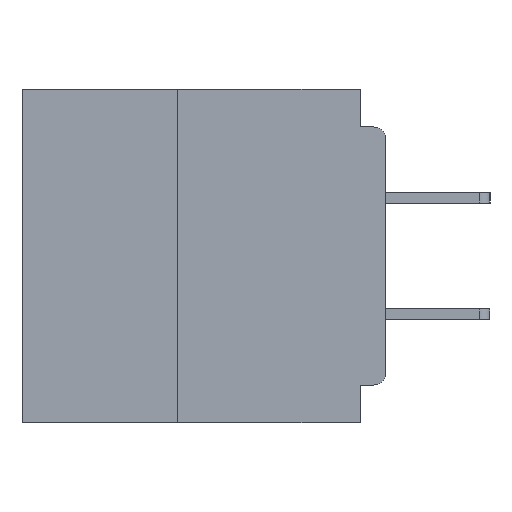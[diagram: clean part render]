
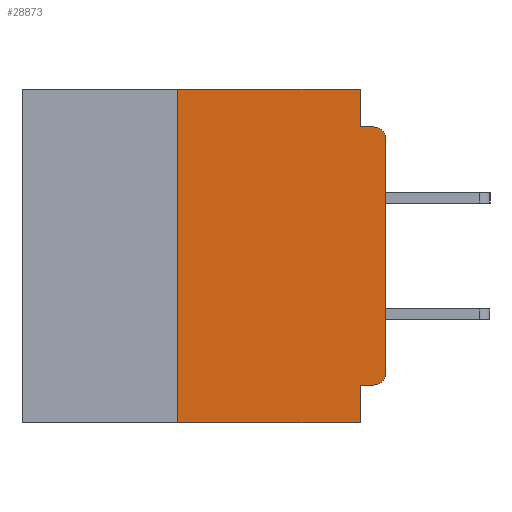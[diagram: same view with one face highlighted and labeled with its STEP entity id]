
A CAD part, left-side view. The second image highlights one B-rep face of the part: STEP entity #28873.
In plain terms, the highlighted planar face has unit normal (-1, 0, 0).
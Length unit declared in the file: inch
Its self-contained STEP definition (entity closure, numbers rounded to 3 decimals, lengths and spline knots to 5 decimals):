
#457 = VECTOR ( 'NONE', #17460, 39.37008 ) ;
#2087 = CARTESIAN_POINT ( 'NONE',  ( 0., 0.25, -0.4 ) ) ;
#2318 = LINE ( 'NONE', #58932, #50608 ) ;
#2635 = VERTEX_POINT ( 'NONE', #54637 ) ;
#4179 = AXIS2_PLACEMENT_3D ( 'NONE', #40658, #12678, #45377 ) ;
#4565 = ORIENTED_EDGE ( 'NONE', *, *, #20370, .T. ) ;
#4714 = LINE ( 'NONE', #22511, #15736 ) ;
#4719 = VERTEX_POINT ( 'NONE', #5902 ) ;
#4881 = LINE ( 'NONE', #22157, #457 ) ;
#5902 = CARTESIAN_POINT ( 'NONE',  ( 0., 0.031, -0.355 ) ) ;
#7995 = CARTESIAN_POINT ( 'NONE',  ( 0., 0.031, 0. ) ) ;
#9453 = ORIENTED_EDGE ( 'NONE', *, *, #44359, .F. ) ;
#9555 = VECTOR ( 'NONE', #11572, 39.37008 ) ;
#9709 = DIRECTION ( 'NONE',  ( -1., 0., 0. ) ) ;
#10058 = LINE ( 'NONE', #37524, #42948 ) ;
#10267 = CARTESIAN_POINT ( 'NONE',  ( 0., 0.031, -0.4 ) ) ;
#10678 = CARTESIAN_POINT ( 'NONE',  ( 0., 0.015, -0.045 ) ) ;
#10918 = DIRECTION ( 'NONE',  ( 0., -1., 0. ) ) ;
#11186 = CARTESIAN_POINT ( 'NONE',  ( 0., 0., -0.34 ) ) ;
#11572 = DIRECTION ( 'NONE',  ( 0., 0., 1. ) ) ;
#11815 = DIRECTION ( 'NONE',  ( 0., 1., 0. ) ) ;
#12678 = DIRECTION ( 'NONE',  ( -1., 0., 0. ) ) ;
#14697 = CIRCLE ( 'NONE', #4179, 0.015 ) ;
#15736 = VECTOR ( 'NONE', #41263, 39.37008 ) ;
#17439 = LINE ( 'NONE', #44492, #54642 ) ;
#17460 = DIRECTION ( 'NONE',  ( 0., -1., 0. ) ) ;
#18369 = DIRECTION ( 'NONE',  ( 1., 0., 0. ) ) ;
#18534 = DIRECTION ( 'NONE',  ( 0., 0., -1. ) ) ;
#19513 = VERTEX_POINT ( 'NONE', #10267 ) ;
#19910 = EDGE_LOOP ( 'NONE', ( #4565, #28558, #40858, #48947, #9453, #22079, #47818, #60266, #43933, #29171 ) ) ;
#20370 = EDGE_CURVE ( 'NONE', #49438, #37737, #2318, .T. ) ;
#22079 = ORIENTED_EDGE ( 'NONE', *, *, #51450, .F. ) ;
#22157 = CARTESIAN_POINT ( 'NONE',  ( 0., 0., -0.045 ) ) ;
#22481 = AXIS2_PLACEMENT_3D ( 'NONE', #37696, #9709, #42407 ) ;
#22511 = CARTESIAN_POINT ( 'NONE',  ( 0., 0.437, 0. ) ) ;
#23654 = VERTEX_POINT ( 'NONE', #10678 ) ;
#24837 = CARTESIAN_POINT ( 'NONE',  ( 0., 0.031, -0.045 ) ) ;
#28186 = EDGE_CURVE ( 'NONE', #37737, #23654, #38001, .T. ) ;
#28558 = ORIENTED_EDGE ( 'NONE', *, *, #28186, .T. ) ;
#28873 = ADVANCED_FACE ( 'NONE', ( #46676 ), #46348, .F. ) ;
#29171 = ORIENTED_EDGE ( 'NONE', *, *, #38684, .T. ) ;
#30952 = VERTEX_POINT ( 'NONE', #34091 ) ;
#30955 = LINE ( 'NONE', #7995, #33883 ) ;
#30957 = VECTOR ( 'NONE', #10918, 39.37008 ) ;
#31080 = DIRECTION ( 'NONE',  ( 0., 0., 1. ) ) ;
#32741 = EDGE_CURVE ( 'NONE', #59971, #19513, #43370, .T. ) ;
#33669 = CARTESIAN_POINT ( 'NONE',  ( 0., 0., -0.06 ) ) ;
#33883 = VECTOR ( 'NONE', #40679, 39.37008 ) ;
#34091 = CARTESIAN_POINT ( 'NONE',  ( 0., 0.25, 0. ) ) ;
#36750 = CARTESIAN_POINT ( 'NONE',  ( 0., 0.437, 0. ) ) ;
#37524 = CARTESIAN_POINT ( 'NONE',  ( 0., 0.031, -0.4 ) ) ;
#37696 = CARTESIAN_POINT ( 'NONE',  ( 0., 0.015, -0.06 ) ) ;
#37737 = VERTEX_POINT ( 'NONE', #33669 ) ;
#38001 = CIRCLE ( 'NONE', #22481, 0.015 ) ;
#38684 = EDGE_CURVE ( 'NONE', #2635, #49438, #14697, .T. ) ;
#40658 = CARTESIAN_POINT ( 'NONE',  ( 0., 0.015, -0.34 ) ) ;
#40679 = DIRECTION ( 'NONE',  ( 0., 0., -1. ) ) ;
#40858 = ORIENTED_EDGE ( 'NONE', *, *, #53920, .F. ) ;
#41263 = DIRECTION ( 'NONE',  ( 0., -1., 0. ) ) ;
#42407 = DIRECTION ( 'NONE',  ( 0., 0., -1. ) ) ;
#42636 = EDGE_CURVE ( 'NONE', #2635, #4719, #17439, .T. ) ;
#42948 = VECTOR ( 'NONE', #18534, 39.37008 ) ;
#43271 = EDGE_CURVE ( 'NONE', #4719, #19513, #10058, .T. ) ;
#43370 = LINE ( 'NONE', #52744, #30957 ) ;
#43933 = ORIENTED_EDGE ( 'NONE', *, *, #42636, .F. ) ;
#44359 = EDGE_CURVE ( 'NONE', #30952, #52330, #4714, .T. ) ;
#44492 = CARTESIAN_POINT ( 'NONE',  ( 0., 0., -0.355 ) ) ;
#45196 = AXIS2_PLACEMENT_3D ( 'NONE', #36750, #18369, #51024 ) ;
#45377 = DIRECTION ( 'NONE',  ( 0., 0., -1. ) ) ;
#46348 = PLANE ( 'NONE',  #45196 ) ;
#46676 = FACE_OUTER_BOUND ( 'NONE', #19910, .T. ) ;
#47665 = CARTESIAN_POINT ( 'NONE',  ( 0., 0.031, 0. ) ) ;
#47818 = ORIENTED_EDGE ( 'NONE', *, *, #32741, .T. ) ;
#48947 = ORIENTED_EDGE ( 'NONE', *, *, #50287, .F. ) ;
#49438 = VERTEX_POINT ( 'NONE', #11186 ) ;
#50287 = EDGE_CURVE ( 'NONE', #52330, #56264, #30955, .T. ) ;
#50608 = VECTOR ( 'NONE', #31080, 39.37008 ) ;
#51024 = DIRECTION ( 'NONE',  ( 0., 0., -1. ) ) ;
#51450 = EDGE_CURVE ( 'NONE', #59971, #30952, #59144, .T. ) ;
#52330 = VERTEX_POINT ( 'NONE', #47665 ) ;
#52744 = CARTESIAN_POINT ( 'NONE',  ( 0., 0.437, -0.4 ) ) ;
#53901 = CARTESIAN_POINT ( 'NONE',  ( 0., 0.25, -0.4 ) ) ;
#53920 = EDGE_CURVE ( 'NONE', #56264, #23654, #4881, .T. ) ;
#54637 = CARTESIAN_POINT ( 'NONE',  ( 0., 0.015, -0.355 ) ) ;
#54642 = VECTOR ( 'NONE', #11815, 39.37008 ) ;
#56264 = VERTEX_POINT ( 'NONE', #24837 ) ;
#58932 = CARTESIAN_POINT ( 'NONE',  ( 0., 0., 0. ) ) ;
#59144 = LINE ( 'NONE', #2087, #9555 ) ;
#59971 = VERTEX_POINT ( 'NONE', #53901 ) ;
#60266 = ORIENTED_EDGE ( 'NONE', *, *, #43271, .F. ) ;
